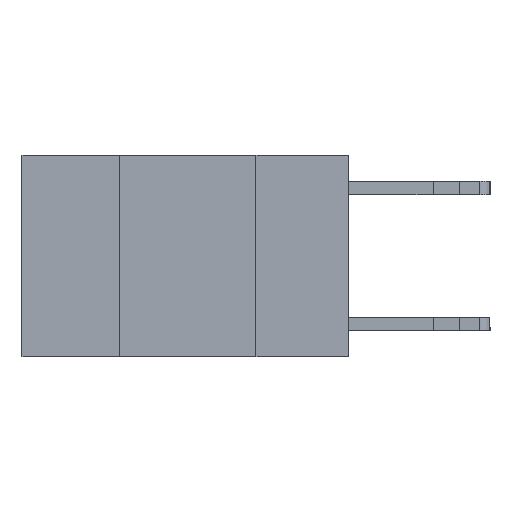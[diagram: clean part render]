
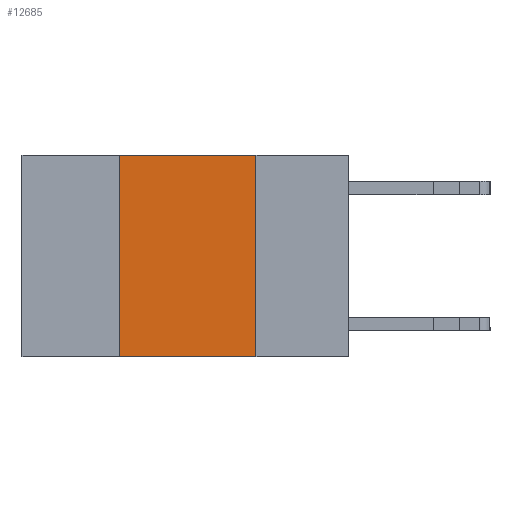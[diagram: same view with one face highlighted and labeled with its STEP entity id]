
A CAD part, left-side view. The second image highlights one B-rep face of the part: STEP entity #12685.
In plain terms, the highlighted planar face has unit normal (-1, 0, 0).
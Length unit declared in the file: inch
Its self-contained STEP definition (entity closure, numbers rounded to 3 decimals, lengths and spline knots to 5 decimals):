
#850 = VERTEX_POINT ( 'NONE', #13078 ) ;
#1207 = EDGE_CURVE ( 'NONE', #11348, #5785, #5984, .T. ) ;
#1253 = DIRECTION ( 'NONE',  ( 0., 0., -1. ) ) ;
#3739 = ORIENTED_EDGE ( 'NONE', *, *, #15168, .F. ) ;
#4426 = CARTESIAN_POINT ( 'NONE',  ( 0., 0.17, -0.37 ) ) ;
#4878 = ORIENTED_EDGE ( 'NONE', *, *, #5545, .F. ) ;
#4908 = DIRECTION ( 'NONE',  ( 0., 0., 1. ) ) ;
#5072 = LINE ( 'NONE', #17128, #12552 ) ;
#5545 = EDGE_CURVE ( 'NONE', #850, #11348, #16884, .T. ) ;
#5785 = VERTEX_POINT ( 'NONE', #10557 ) ;
#5984 = LINE ( 'NONE', #10080, #8309 ) ;
#6360 = ORIENTED_EDGE ( 'NONE', *, *, #1207, .F. ) ;
#6362 = CARTESIAN_POINT ( 'NONE',  ( 0., 0.6, 0. ) ) ;
#6542 = ORIENTED_EDGE ( 'NONE', *, *, #10223, .T. ) ;
#6545 = PLANE ( 'NONE',  #11693 ) ;
#7741 = VECTOR ( 'NONE', #12609, 39.37008 ) ;
#8309 = VECTOR ( 'NONE', #11309, 39.37008 ) ;
#8459 = EDGE_LOOP ( 'NONE', ( #3739, #6360, #4878, #6542 ) ) ;
#8747 = CARTESIAN_POINT ( 'NONE',  ( 0., 0.42, 0. ) ) ;
#10080 = CARTESIAN_POINT ( 'NONE',  ( 0., 0.6, 0. ) ) ;
#10223 = EDGE_CURVE ( 'NONE', #850, #10375, #5072, .T. ) ;
#10375 = VERTEX_POINT ( 'NONE', #4426 ) ;
#10557 = CARTESIAN_POINT ( 'NONE',  ( 0., 0.17, 0. ) ) ;
#11309 = DIRECTION ( 'NONE',  ( 0., -1., 0. ) ) ;
#11348 = VERTEX_POINT ( 'NONE', #16933 ) ;
#11687 = DIRECTION ( 'NONE',  ( 1., 0., 0. ) ) ;
#11693 = AXIS2_PLACEMENT_3D ( 'NONE', #6362, #11687, #1253 ) ;
#12505 = LINE ( 'NONE', #16559, #7741 ) ;
#12552 = VECTOR ( 'NONE', #17212, 39.37008 ) ;
#12609 = DIRECTION ( 'NONE',  ( 0., 0., -1. ) ) ;
#12685 = ADVANCED_FACE ( 'NONE', ( #13094 ), #6545, .F. ) ;
#13078 = CARTESIAN_POINT ( 'NONE',  ( 0., 0.42, -0.37 ) ) ;
#13094 = FACE_OUTER_BOUND ( 'NONE', #8459, .T. ) ;
#15168 = EDGE_CURVE ( 'NONE', #5785, #10375, #12505, .T. ) ;
#16559 = CARTESIAN_POINT ( 'NONE',  ( 0., 0.17, 0. ) ) ;
#16884 = LINE ( 'NONE', #8747, #17074 ) ;
#16933 = CARTESIAN_POINT ( 'NONE',  ( 0., 0.42, 0. ) ) ;
#17074 = VECTOR ( 'NONE', #4908, 39.37008 ) ;
#17128 = CARTESIAN_POINT ( 'NONE',  ( 0., 0.6, -0.37 ) ) ;
#17212 = DIRECTION ( 'NONE',  ( 0., -1., 0. ) ) ;
